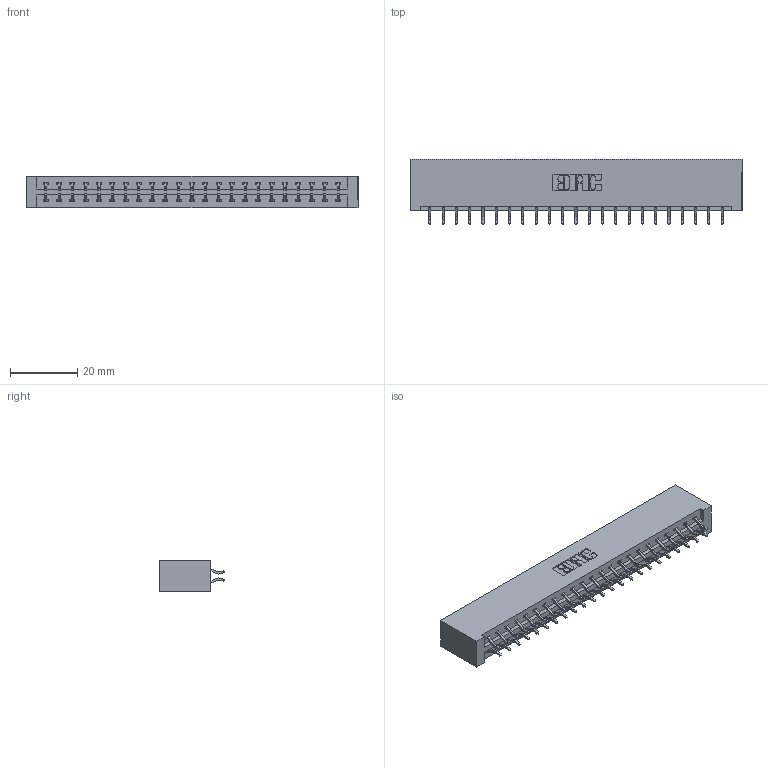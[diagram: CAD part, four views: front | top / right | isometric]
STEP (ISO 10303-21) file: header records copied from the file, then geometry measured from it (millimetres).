
FILE_DESCRIPTION (( 'STEP AP203' ), '1' );
FILE_NAME ('387-046-556-201.STEP', '2019-10-18T08:15:01', ( '' ), ( '' ), 'SwSTEP 2.0', 'SolidWorks 2016', '' );
FILE_SCHEMA (( 'CONFIG_CONTROL_DESIGN' ));
Length unit declared in the file: inch
Products named in the file (3): 387-046-556-201; 337 Part_No Mounting Lugs; 345-292-001_556 Tail
Assembly tree (47 placements, depth 2):
  387-046-556-201
    337 Part_No Mounting Lugs
    345-292-001_556 Tail  x46
Bounding box: 99.01 x 19.57 x 9.4 mm (x, y, z)
Volume: 10940.4 mm3; surface area: 12191.1 mm2
Topology: 47 solids, 47 shells, 2866 faces, 8521 edges, 5618 vertices
Faces by surface type: plane 1998, cylinder 868
Entity records: 20233 total; most frequent: CARTESIAN_POINT 3438, ORIENTED_EDGE 3362, DIRECTION 2941, EDGE_CURVE 1681, LINE 1553, VECTOR 1553, VERTEX_POINT 1118, AXIS2_PLACEMENT_3D 694
